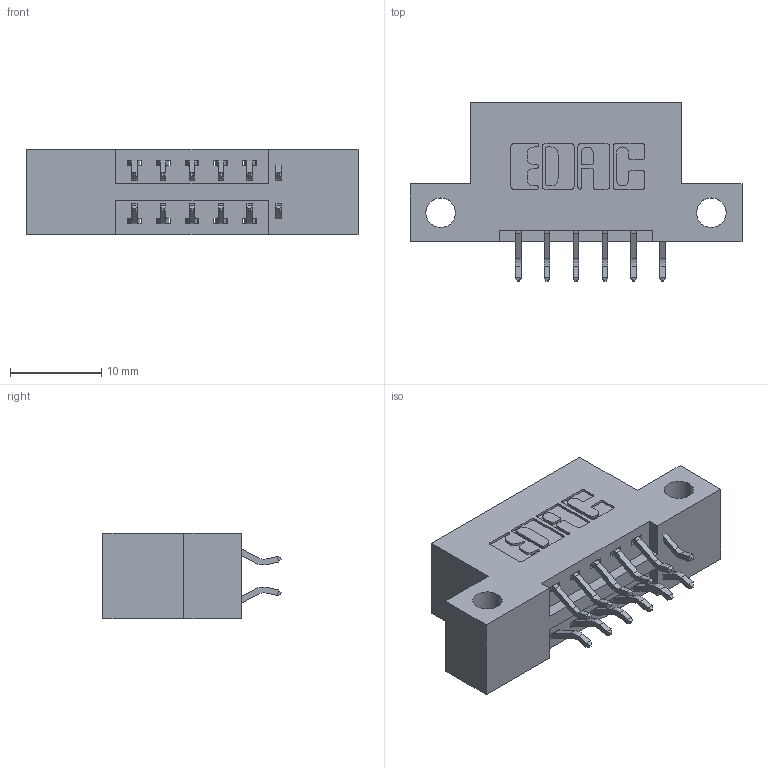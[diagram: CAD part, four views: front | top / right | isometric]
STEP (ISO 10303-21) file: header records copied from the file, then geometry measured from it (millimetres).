
FILE_DESCRIPTION (( 'STEP AP203' ), '1' );
FILE_NAME ('346-012-556-212.STEP', '2022-05-17T20:34:23', ( '' ), ( '' ), 'SwSTEP 2.0', 'SolidWorks 2020', '' );
FILE_SCHEMA (( 'CONFIG_CONTROL_DESIGN' ));
Length unit declared in the file: inch
Products named in the file (3): 346 Part_Flush Mounting Lugs - Side Mount; 345-292-001_556 Tail; 346-012-556-212
Assembly tree (13 placements, depth 2):
  346-012-556-212
    346 Part_Flush Mounting Lugs - Side Mount
    345-292-001_556 Tail  x12
Bounding box: 36.45 x 19.57 x 9.4 mm (x, y, z)
Volume: 3197.1 mm3; surface area: 3768.3 mm2
Topology: 13 solids, 13 shells, 806 faces, 2363 edges, 1558 vertices
Faces by surface type: plane 534, cylinder 272
Entity records: 8531 total; most frequent: CARTESIAN_POINT 1462, ORIENTED_EDGE 1382, DIRECTION 1331, EDGE_CURVE 691, VECTOR 531, LINE 531, VERTEX_POINT 458, AXIS2_PLACEMENT_3D 400
